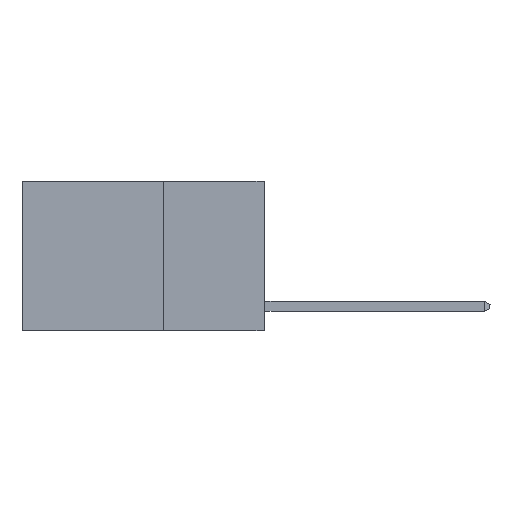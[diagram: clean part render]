
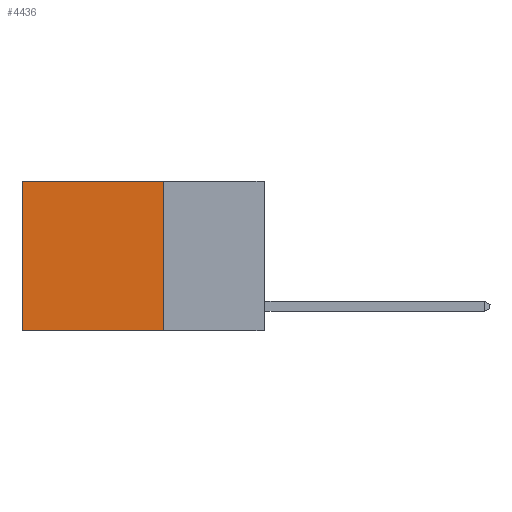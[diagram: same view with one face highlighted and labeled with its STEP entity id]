
A CAD part, left-side view. The second image highlights one B-rep face of the part: STEP entity #4436.
In plain terms, the highlighted planar face has unit normal (-1, 0, 0).
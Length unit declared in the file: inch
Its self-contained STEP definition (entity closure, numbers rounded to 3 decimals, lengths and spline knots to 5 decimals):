
#465 = LINE ( 'NONE', #20638, #1020 ) ;
#696 = VECTOR ( 'NONE', #1909, 39.37008 ) ;
#1002 = DIRECTION ( 'NONE',  ( 0., 0., -1. ) ) ;
#1020 = VECTOR ( 'NONE', #2281, 39.37008 ) ;
#1077 = CARTESIAN_POINT ( 'NONE',  ( 0.2625, 0.25, -0.37 ) ) ;
#1909 = DIRECTION ( 'NONE',  ( 0., 1., 0. ) ) ;
#2207 = EDGE_CURVE ( 'NONE', #20287, #19366, #21871, .T. ) ;
#2281 = DIRECTION ( 'NONE',  ( 0., 0., -1. ) ) ;
#3335 = VERTEX_POINT ( 'NONE', #23229 ) ;
#3884 = EDGE_CURVE ( 'NONE', #3335, #20287, #16678, .T. ) ;
#4185 = CARTESIAN_POINT ( 'NONE',  ( 0.2625, 0.25, 0. ) ) ;
#4436 = ADVANCED_FACE ( 'NONE', ( #21793 ), #12230, .F. ) ;
#4875 = AXIS2_PLACEMENT_3D ( 'NONE', #9952, #19195, #1002 ) ;
#6011 = VERTEX_POINT ( 'NONE', #14292 ) ;
#6816 = ORIENTED_EDGE ( 'NONE', *, *, #3884, .F. ) ;
#9952 = CARTESIAN_POINT ( 'NONE',  ( 0.2625, 0.25, 0. ) ) ;
#12230 = PLANE ( 'NONE',  #4875 ) ;
#14292 = CARTESIAN_POINT ( 'NONE',  ( 0.2625, 0.6, 0. ) ) ;
#15050 = VECTOR ( 'NONE', #19397, 39.37008 ) ;
#15727 = LINE ( 'NONE', #4185, #696 ) ;
#16678 = LINE ( 'NONE', #21683, #15050 ) ;
#17568 = EDGE_CURVE ( 'NONE', #3335, #6011, #15727, .T. ) ;
#18819 = CARTESIAN_POINT ( 'NONE',  ( 0.2625, 0.6, -0.37 ) ) ;
#19195 = DIRECTION ( 'NONE',  ( 1., 0., 0. ) ) ;
#19366 = VERTEX_POINT ( 'NONE', #18819 ) ;
#19397 = DIRECTION ( 'NONE',  ( 0., 0., -1. ) ) ;
#20287 = VERTEX_POINT ( 'NONE', #22997 ) ;
#20638 = CARTESIAN_POINT ( 'NONE',  ( 0.2625, 0.6, 0. ) ) ;
#21683 = CARTESIAN_POINT ( 'NONE',  ( 0.2625, 0.25, 0. ) ) ;
#21793 = FACE_OUTER_BOUND ( 'NONE', #24857, .T. ) ;
#21871 = LINE ( 'NONE', #1077, #27505 ) ;
#22997 = CARTESIAN_POINT ( 'NONE',  ( 0.2625, 0.25, -0.37 ) ) ;
#23229 = CARTESIAN_POINT ( 'NONE',  ( 0.2625, 0.25, 0. ) ) ;
#24857 = EDGE_LOOP ( 'NONE', ( #28070, #29007, #6816, #27351 ) ) ;
#26490 = EDGE_CURVE ( 'NONE', #6011, #19366, #465, .T. ) ;
#27351 = ORIENTED_EDGE ( 'NONE', *, *, #17568, .T. ) ;
#27505 = VECTOR ( 'NONE', #28835, 39.37008 ) ;
#28070 = ORIENTED_EDGE ( 'NONE', *, *, #26490, .T. ) ;
#28835 = DIRECTION ( 'NONE',  ( 0., 1., 0. ) ) ;
#29007 = ORIENTED_EDGE ( 'NONE', *, *, #2207, .F. ) ;
